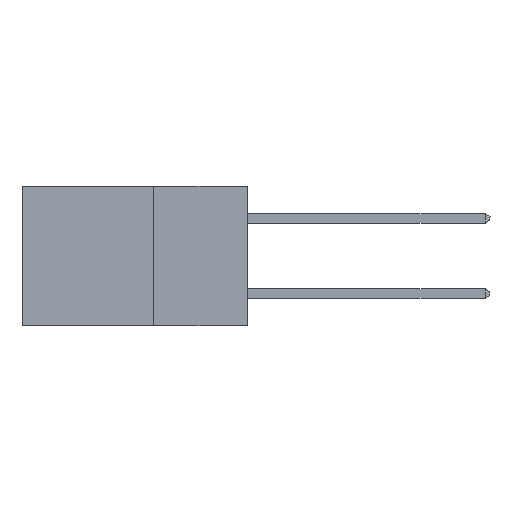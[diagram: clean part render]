
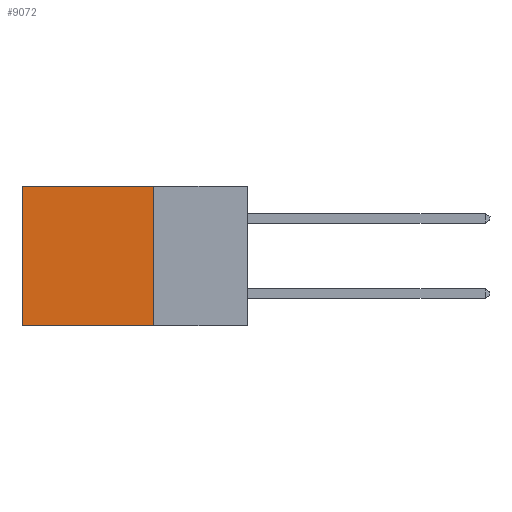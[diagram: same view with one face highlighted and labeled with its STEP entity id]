
A CAD part, left-side view. The second image highlights one B-rep face of the part: STEP entity #9072.
In plain terms, the highlighted planar face has unit normal (-1, 0, 0).
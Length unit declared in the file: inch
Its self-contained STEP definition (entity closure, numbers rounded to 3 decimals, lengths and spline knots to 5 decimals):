
#473 = CARTESIAN_POINT ( 'NONE',  ( 0.2615, 0.25, 0. ) ) ;
#599 = VECTOR ( 'NONE', #10430, 39.37008 ) ;
#807 = ORIENTED_EDGE ( 'NONE', *, *, #5405, .F. ) ;
#1557 = EDGE_CURVE ( 'NONE', #3337, #10061, #10589, .T. ) ;
#1749 = DIRECTION ( 'NONE',  ( 0., 1., 0. ) ) ;
#1882 = CARTESIAN_POINT ( 'NONE',  ( 0.2615, 0.6, 0. ) ) ;
#2314 = VERTEX_POINT ( 'NONE', #6830 ) ;
#2428 = EDGE_LOOP ( 'NONE', ( #8745, #807, #3047, #5324 ) ) ;
#2835 = CARTESIAN_POINT ( 'NONE',  ( 0.2615, 0.25, -0.37 ) ) ;
#3047 = ORIENTED_EDGE ( 'NONE', *, *, #5344, .F. ) ;
#3095 = CARTESIAN_POINT ( 'NONE',  ( 0.2615, 0.25, 0. ) ) ;
#3337 = VERTEX_POINT ( 'NONE', #473 ) ;
#4216 = DIRECTION ( 'NONE',  ( 0., 0., -1. ) ) ;
#4386 = DIRECTION ( 'NONE',  ( 1., 0., 0. ) ) ;
#4639 = EDGE_CURVE ( 'NONE', #10061, #2314, #7079, .T. ) ;
#5161 = FACE_OUTER_BOUND ( 'NONE', #2428, .T. ) ;
#5324 = ORIENTED_EDGE ( 'NONE', *, *, #1557, .T. ) ;
#5344 = EDGE_CURVE ( 'NONE', #3337, #6328, #9977, .T. ) ;
#5378 = CARTESIAN_POINT ( 'NONE',  ( 0.2615, 0.6, -0.37 ) ) ;
#5405 = EDGE_CURVE ( 'NONE', #6328, #2314, #8424, .T. ) ;
#5582 = AXIS2_PLACEMENT_3D ( 'NONE', #2835, #4386, #7665 ) ;
#6224 = VECTOR ( 'NONE', #1749, 39.37008 ) ;
#6328 = VERTEX_POINT ( 'NONE', #9140 ) ;
#6800 = PLANE ( 'NONE',  #5582 ) ;
#6830 = CARTESIAN_POINT ( 'NONE',  ( 0.2615, 0.6, -0.37 ) ) ;
#7079 = LINE ( 'NONE', #5378, #599 ) ;
#7584 = CARTESIAN_POINT ( 'NONE',  ( 0.2615, 0.25, -0.37 ) ) ;
#7665 = DIRECTION ( 'NONE',  ( 0., 0., -1. ) ) ;
#8424 = LINE ( 'NONE', #9138, #6224 ) ;
#8745 = ORIENTED_EDGE ( 'NONE', *, *, #4639, .T. ) ;
#9072 = ADVANCED_FACE ( 'NONE', ( #5161 ), #6800, .F. ) ;
#9138 = CARTESIAN_POINT ( 'NONE',  ( 0.2615, 0.25, -0.37 ) ) ;
#9140 = CARTESIAN_POINT ( 'NONE',  ( 0.2615, 0.25, -0.37 ) ) ;
#9377 = VECTOR ( 'NONE', #4216, 39.37008 ) ;
#9768 = DIRECTION ( 'NONE',  ( 0., 1., 0. ) ) ;
#9977 = LINE ( 'NONE', #7584, #9377 ) ;
#10061 = VERTEX_POINT ( 'NONE', #1882 ) ;
#10430 = DIRECTION ( 'NONE',  ( 0., 0., -1. ) ) ;
#10589 = LINE ( 'NONE', #3095, #10604 ) ;
#10604 = VECTOR ( 'NONE', #9768, 39.37008 ) ;
